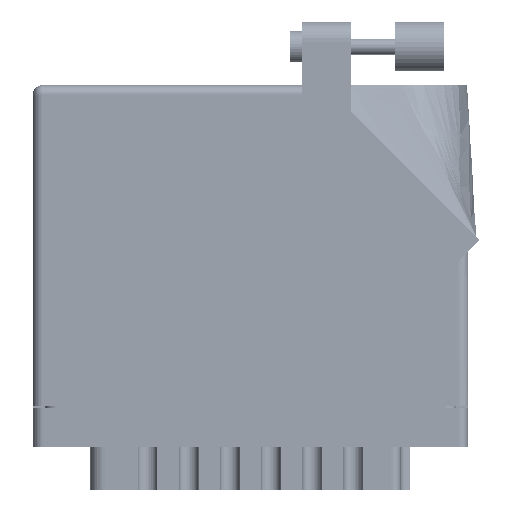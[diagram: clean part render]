
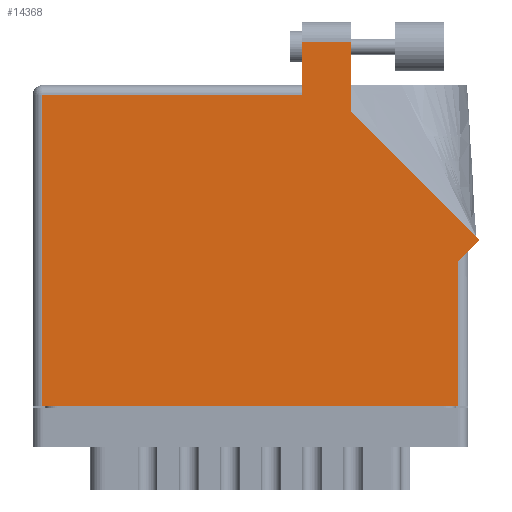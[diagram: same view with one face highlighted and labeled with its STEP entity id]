
A CAD part, front view. The second image highlights one B-rep face of the part: STEP entity #14368.
In plain terms, the highlighted face is planar.
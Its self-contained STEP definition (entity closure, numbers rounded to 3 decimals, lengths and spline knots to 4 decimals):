
#781 = DIRECTION ( 'NONE',  ( 0., 1., 0. ) ) ;
#803 = DIRECTION ( 'NONE',  ( -1., 0., 0. ) ) ;
#1887 = EDGE_CURVE ( 'NONE', #75145, #31136, #41698, .T. ) ;
#2243 = VECTOR ( 'NONE', #781, 39.3701 ) ;
#4006 = CARTESIAN_POINT ( 'NONE',  ( 0., 0., 0. ) ) ;
#4011 = LINE ( 'NONE', #37277, #36582 ) ;
#5702 = DIRECTION ( 'NONE',  ( 0., -1., 0. ) ) ;
#6638 = AXIS2_PLACEMENT_3D ( 'NONE', #69365, #11602, #84067 ) ;
#6644 = VECTOR ( 'NONE', #30306, 39.3701 ) ;
#7073 = VERTEX_POINT ( 'NONE', #65684 ) ;
#7088 = CARTESIAN_POINT ( 'NONE',  ( 2.012, 1.8644, 0. ) ) ;
#9229 = CARTESIAN_POINT ( 'NONE',  ( 2.755, 0.98, 0. ) ) ;
#10229 = VERTEX_POINT ( 'NONE', #26709 ) ;
#11602 = DIRECTION ( 'NONE',  ( 0., 0., -1. ) ) ;
#13529 = CARTESIAN_POINT ( 'NONE',  ( 2.693, 0.918, 0. ) ) ;
#14368 = ADVANCED_FACE ( 'NONE', ( #53099 ), #54605, .F. ) ;
#15214 = CARTESIAN_POINT ( 'NONE',  ( 2.693, 0.98, 0. ) ) ;
#17661 = ORIENTED_EDGE ( 'NONE', *, *, #40422, .T. ) ;
#18756 = EDGE_CURVE ( 'NONE', #61619, #80791, #80566, .T. ) ;
#20145 = EDGE_CURVE ( 'NONE', #7073, #36003, #78994, .T. ) ;
#23977 = DIRECTION ( 'NONE',  ( -0.707, 0.707, 0. ) ) ;
#26017 = VECTOR ( 'NONE', #44736, 39.3701 ) ;
#26709 = CARTESIAN_POINT ( 'NONE',  ( 2.012, 1.8644, 0. ) ) ;
#28514 = CARTESIAN_POINT ( 'NONE',  ( 2.693, 0., 0. ) ) ;
#30306 = DIRECTION ( 'NONE',  ( 0., 1., 0. ) ) ;
#30508 = ORIENTED_EDGE ( 'NONE', *, *, #1887, .T. ) ;
#31136 = VERTEX_POINT ( 'NONE', #50242 ) ;
#32803 = ORIENTED_EDGE ( 'NONE', *, *, #18756, .T. ) ;
#36003 = VERTEX_POINT ( 'NONE', #43192 ) ;
#36582 = VECTOR ( 'NONE', #80230, 39.3701 ) ;
#37277 = CARTESIAN_POINT ( 'NONE',  ( 0.062, 0., 0. ) ) ;
#40422 = EDGE_CURVE ( 'NONE', #80791, #7073, #83841, .T. ) ;
#41698 = LINE ( 'NONE', #9229, #26017 ) ;
#42586 = EDGE_CURVE ( 'NONE', #31136, #10229, #82270, .T. ) ;
#43192 = CARTESIAN_POINT ( 'NONE',  ( 0.062, 1.968, 0. ) ) ;
#44736 = DIRECTION ( 'NONE',  ( 0.707, 0.707, 0. ) ) ;
#44847 = EDGE_CURVE ( 'NONE', #10229, #61619, #70914, .T. ) ;
#45285 = LINE ( 'NONE', #4006, #65545 ) ;
#47044 = DIRECTION ( 'NONE',  ( 1., 0., 0. ) ) ;
#49715 = ORIENTED_EDGE ( 'NONE', *, *, #67778, .T. ) ;
#50242 = CARTESIAN_POINT ( 'NONE',  ( 2.8257, 1.0507, 0. ) ) ;
#50858 = EDGE_CURVE ( 'NONE', #36003, #66458, #4011, .T. ) ;
#53099 = FACE_OUTER_BOUND ( 'NONE', #53765, .T. ) ;
#53566 = CARTESIAN_POINT ( 'NONE',  ( 2.012, 2.305, 0. ) ) ;
#53765 = EDGE_LOOP ( 'NONE', ( #84410, #32803, #17661, #61783, #75693, #49715, #87441, #30508, #73830 ) ) ;
#54316 = DIRECTION ( 'NONE',  ( -1., 0., 0. ) ) ;
#54605 = PLANE ( 'NONE',  #6638 ) ;
#56387 = VECTOR ( 'NONE', #23977, 39.3701 ) ;
#61619 = VERTEX_POINT ( 'NONE', #53566 ) ;
#61783 = ORIENTED_EDGE ( 'NONE', *, *, #20145, .T. ) ;
#62259 = CARTESIAN_POINT ( 'NONE',  ( 1.705, 2.03, 0. ) ) ;
#62524 = VECTOR ( 'NONE', #5702, 39.3701 ) ;
#65545 = VECTOR ( 'NONE', #47044, 39.3701 ) ;
#65684 = CARTESIAN_POINT ( 'NONE',  ( 1.705, 1.968, 0. ) ) ;
#66458 = VERTEX_POINT ( 'NONE', #73312 ) ;
#67778 = EDGE_CURVE ( 'NONE', #66458, #82366, #45285, .T. ) ;
#69365 = CARTESIAN_POINT ( 'NONE',  ( 0., 2.03, 0. ) ) ;
#70914 = LINE ( 'NONE', #7088, #2243 ) ;
#71496 = CARTESIAN_POINT ( 'NONE',  ( 0., 1.968, 0. ) ) ;
#73312 = CARTESIAN_POINT ( 'NONE',  ( 0.062, 0., 0. ) ) ;
#73830 = ORIENTED_EDGE ( 'NONE', *, *, #42586, .T. ) ;
#74670 = EDGE_CURVE ( 'NONE', #82366, #75145, #79726, .T. ) ;
#75145 = VERTEX_POINT ( 'NONE', #13529 ) ;
#75693 = ORIENTED_EDGE ( 'NONE', *, *, #50858, .T. ) ;
#76551 = CARTESIAN_POINT ( 'NONE',  ( 1.705, 2.305, 0. ) ) ;
#78885 = VECTOR ( 'NONE', #803, 39.3701 ) ;
#78994 = LINE ( 'NONE', #71496, #78885 ) ;
#79726 = LINE ( 'NONE', #15214, #6644 ) ;
#80230 = DIRECTION ( 'NONE',  ( 0., -1., 0. ) ) ;
#80500 = CARTESIAN_POINT ( 'NONE',  ( 1.705, 2.305, 0. ) ) ;
#80566 = LINE ( 'NONE', #76551, #90690 ) ;
#80791 = VERTEX_POINT ( 'NONE', #80500 ) ;
#81343 = CARTESIAN_POINT ( 'NONE',  ( 2.8257, 1.0507, 0. ) ) ;
#82270 = LINE ( 'NONE', #81343, #56387 ) ;
#82366 = VERTEX_POINT ( 'NONE', #28514 ) ;
#83841 = LINE ( 'NONE', #62259, #62524 ) ;
#84067 = DIRECTION ( 'NONE',  ( -1., 0., 0. ) ) ;
#84410 = ORIENTED_EDGE ( 'NONE', *, *, #44847, .T. ) ;
#87441 = ORIENTED_EDGE ( 'NONE', *, *, #74670, .T. ) ;
#90690 = VECTOR ( 'NONE', #54316, 39.3701 ) ;
